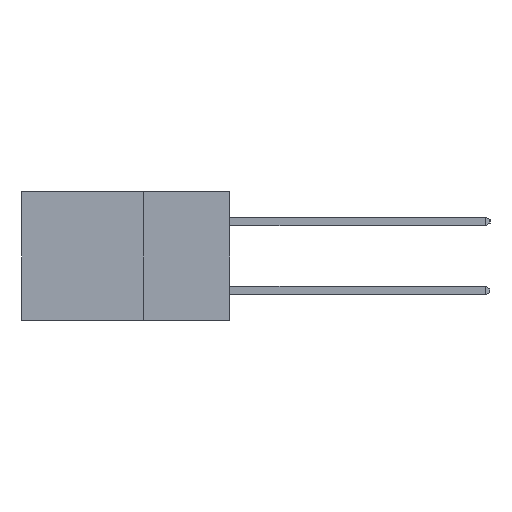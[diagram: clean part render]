
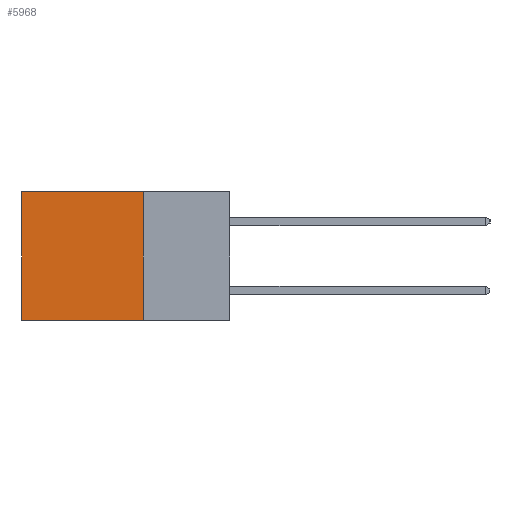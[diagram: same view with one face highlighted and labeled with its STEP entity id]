
A CAD part, left-side view. The second image highlights one B-rep face of the part: STEP entity #5968.
In plain terms, the highlighted planar face has unit normal (-1, 0, 0).
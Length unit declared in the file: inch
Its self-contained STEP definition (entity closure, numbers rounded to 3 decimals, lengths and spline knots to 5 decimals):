
#1831 = CARTESIAN_POINT ( 'NONE',  ( 0.2615, 0.25, -0.37 ) ) ;
#2364 = VERTEX_POINT ( 'NONE', #19285 ) ;
#3838 = EDGE_CURVE ( 'NONE', #2364, #9778, #7781, .T. ) ;
#4148 = VERTEX_POINT ( 'NONE', #20449 ) ;
#4726 = ORIENTED_EDGE ( 'NONE', *, *, #20713, .T. ) ;
#4728 = EDGE_CURVE ( 'NONE', #9778, #13834, #6476, .T. ) ;
#4893 = DIRECTION ( 'NONE',  ( 1., 0., 0. ) ) ;
#5968 = ADVANCED_FACE ( 'NONE', ( #25022 ), #10956, .F. ) ;
#6476 = LINE ( 'NONE', #1831, #16564 ) ;
#7327 = ORIENTED_EDGE ( 'NONE', *, *, #4728, .F. ) ;
#7717 = LINE ( 'NONE', #13781, #17188 ) ;
#7781 = LINE ( 'NONE', #22393, #12544 ) ;
#9554 = CARTESIAN_POINT ( 'NONE',  ( 0.2615, 0.6, -0.37 ) ) ;
#9778 = VERTEX_POINT ( 'NONE', #22909 ) ;
#10956 = PLANE ( 'NONE',  #17584 ) ;
#11857 = DIRECTION ( 'NONE',  ( 0., 1., 0. ) ) ;
#12544 = VECTOR ( 'NONE', #22417, 39.37008 ) ;
#13305 = EDGE_CURVE ( 'NONE', #2364, #4148, #7717, .T. ) ;
#13781 = CARTESIAN_POINT ( 'NONE',  ( 0.2615, 0.25, 0. ) ) ;
#13834 = VERTEX_POINT ( 'NONE', #9554 ) ;
#14605 = CARTESIAN_POINT ( 'NONE',  ( 0.2615, 0.6, -0.37 ) ) ;
#14660 = EDGE_LOOP ( 'NONE', ( #4726, #7327, #17093, #15931 ) ) ;
#15931 = ORIENTED_EDGE ( 'NONE', *, *, #13305, .T. ) ;
#16051 = LINE ( 'NONE', #14605, #16671 ) ;
#16564 = VECTOR ( 'NONE', #17037, 39.37008 ) ;
#16614 = DIRECTION ( 'NONE',  ( 0., 0., -1. ) ) ;
#16671 = VECTOR ( 'NONE', #16614, 39.37008 ) ;
#16999 = CARTESIAN_POINT ( 'NONE',  ( 0.2615, 0.25, -0.37 ) ) ;
#17037 = DIRECTION ( 'NONE',  ( 0., 1., 0. ) ) ;
#17093 = ORIENTED_EDGE ( 'NONE', *, *, #3838, .F. ) ;
#17188 = VECTOR ( 'NONE', #11857, 39.37008 ) ;
#17584 = AXIS2_PLACEMENT_3D ( 'NONE', #16999, #4893, #19031 ) ;
#19031 = DIRECTION ( 'NONE',  ( 0., 0., -1. ) ) ;
#19285 = CARTESIAN_POINT ( 'NONE',  ( 0.2615, 0.25, 0. ) ) ;
#20449 = CARTESIAN_POINT ( 'NONE',  ( 0.2615, 0.6, 0. ) ) ;
#20713 = EDGE_CURVE ( 'NONE', #4148, #13834, #16051, .T. ) ;
#22393 = CARTESIAN_POINT ( 'NONE',  ( 0.2615, 0.25, -0.37 ) ) ;
#22417 = DIRECTION ( 'NONE',  ( 0., 0., -1. ) ) ;
#22909 = CARTESIAN_POINT ( 'NONE',  ( 0.2615, 0.25, -0.37 ) ) ;
#25022 = FACE_OUTER_BOUND ( 'NONE', #14660, .T. ) ;
